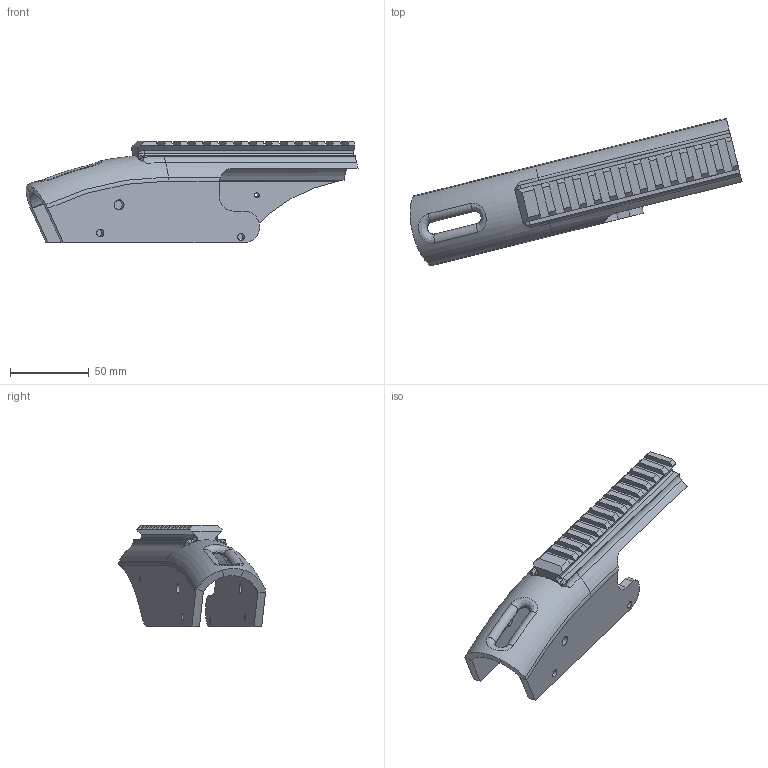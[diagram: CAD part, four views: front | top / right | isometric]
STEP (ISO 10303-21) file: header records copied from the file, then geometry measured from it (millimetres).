
FILE_DESCRIPTION(/* description */ (''),/* implementation_level */ '2;1');
FILE_NAME(/* name */ 'MOSSBERG.RAIL.stp',/* time_stamp */ '2014-10-01T18:10:08+02:00',/* author */ ('parasporo'),/* organization */ (''),/* preprocessor_version */ 'ST-DEVELOPER v15.2',/* originating_system */ 'Autodesk Inventor LT ',/* authorisation */ '');
FILE_SCHEMA (('AUTOMOTIVE_DESIGN { 1 0 10303 214 3 1 1 }'));
Length unit declared in the file: millimetre
Products named in the file (1): Mill 500 .2assembly
Bounding box: 210.71 x 93.39 x 64.61 mm (x, y, z)
Volume: 120972.7 mm3; surface area: 49122.6 mm2
Topology: 1 solids, 1 shells, 227 faces, 663 edges, 434 vertices
Faces by surface type: plane 125, bspline 57, cylinder 29, torus 12, cone 4
Full cylindrical faces by diameter (mm): 3.1 x1, 4.55 x1, 4.75 x2, 6.32 x2
Entity records: 27937 total; most frequent: CARTESIAN_POINT 22339, ORIENTED_EDGE 1302, DIRECTION 926, EDGE_CURVE 651, VERTEX_POINT 428, LINE 398, VECTOR 398, AXIS2_PLACEMENT_3D 264
